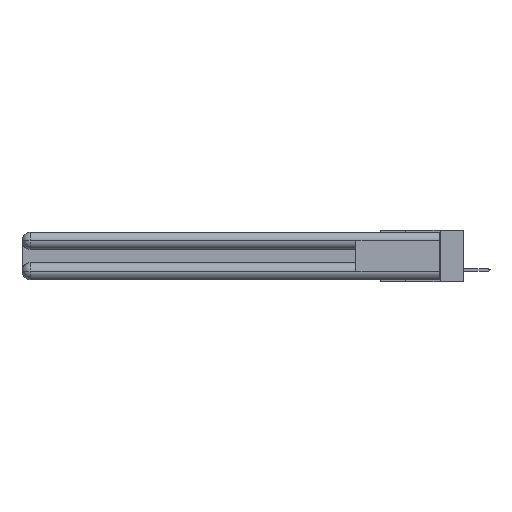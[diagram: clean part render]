
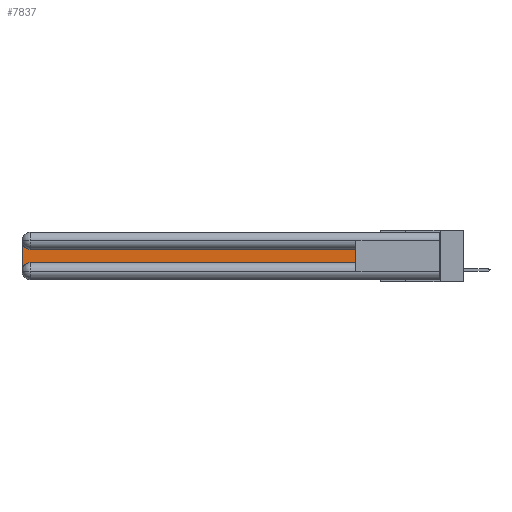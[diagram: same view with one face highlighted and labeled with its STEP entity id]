
A CAD part, left-side view. The second image highlights one B-rep face of the part: STEP entity #7837.
In plain terms, the highlighted planar face has unit normal (-1, 0, 0).
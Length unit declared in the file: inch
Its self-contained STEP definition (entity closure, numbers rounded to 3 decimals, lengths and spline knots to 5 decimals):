
#188 = EDGE_CURVE ( 'NONE', #23155, #506, #2117, .T. ) ;
#506 = VERTEX_POINT ( 'NONE', #878 ) ;
#878 = CARTESIAN_POINT ( 'NONE',  ( 0.075, 2.94, -0.2175 ) ) ;
#973 = CARTESIAN_POINT ( 'NONE',  ( 0.075, 0.6, -0.1225 ) ) ;
#992 = FACE_OUTER_BOUND ( 'NONE', #26921, .T. ) ;
#1017 = AXIS2_PLACEMENT_3D ( 'NONE', #15158, #3985, #22976 ) ;
#1837 = ORIENTED_EDGE ( 'NONE', *, *, #188, .T. ) ;
#2117 = CIRCLE ( 'NONE', #8973, 0.06 ) ;
#2458 = ORIENTED_EDGE ( 'NONE', *, *, #16512, .T. ) ;
#3915 = LINE ( 'NONE', #973, #23005 ) ;
#3985 = DIRECTION ( 'NONE',  ( 1., 0., 0. ) ) ;
#4199 = CIRCLE ( 'NONE', #1017, 0.06 ) ;
#5068 = CARTESIAN_POINT ( 'NONE',  ( 0.075, 0.6, -0.2175 ) ) ;
#6595 = CARTESIAN_POINT ( 'NONE',  ( 0.075, 3., -0.2175 ) ) ;
#7837 = ADVANCED_FACE ( 'NONE', ( #992 ), #11448, .F. ) ;
#8078 = AXIS2_PLACEMENT_3D ( 'NONE', #23175, #27730, #20929 ) ;
#8739 = VERTEX_POINT ( 'NONE', #21178 ) ;
#8973 = AXIS2_PLACEMENT_3D ( 'NONE', #25757, #11678, #11375 ) ;
#9025 = CARTESIAN_POINT ( 'NONE',  ( 0.075, 0.6, -0.1225 ) ) ;
#9515 = EDGE_CURVE ( 'NONE', #15710, #8739, #4199, .T. ) ;
#9589 = ORIENTED_EDGE ( 'NONE', *, *, #11261, .T. ) ;
#11261 = EDGE_CURVE ( 'NONE', #8739, #23155, #26998, .T. ) ;
#11375 = DIRECTION ( 'NONE',  ( 0., 0., -1. ) ) ;
#11448 = PLANE ( 'NONE',  #8078 ) ;
#11678 = DIRECTION ( 'NONE',  ( 1., 0., 0. ) ) ;
#12308 = ORIENTED_EDGE ( 'NONE', *, *, #24619, .T. ) ;
#13381 = CARTESIAN_POINT ( 'NONE',  ( 0.075, 2.94, -0.1225 ) ) ;
#13755 = VECTOR ( 'NONE', #20746, 39.37008 ) ;
#13794 = VECTOR ( 'NONE', #29493, 39.37008 ) ;
#14466 = VERTEX_POINT ( 'NONE', #5068 ) ;
#15158 = CARTESIAN_POINT ( 'NONE',  ( 0.075, 2.94, -0.0625 ) ) ;
#15416 = CARTESIAN_POINT ( 'NONE',  ( 0.075, 0.6, -0.2175 ) ) ;
#15710 = VERTEX_POINT ( 'NONE', #13381 ) ;
#15789 = ORIENTED_EDGE ( 'NONE', *, *, #26284, .T. ) ;
#16512 = EDGE_CURVE ( 'NONE', #14466, #16564, #20800, .T. ) ;
#16564 = VERTEX_POINT ( 'NONE', #9025 ) ;
#19490 = CARTESIAN_POINT ( 'NONE',  ( 0.075, 0.6, -0.2175 ) ) ;
#19597 = VECTOR ( 'NONE', #26778, 39.37008 ) ;
#19760 = DIRECTION ( 'NONE',  ( 0., 1., 0. ) ) ;
#20746 = DIRECTION ( 'NONE',  ( 0., 0., -1. ) ) ;
#20800 = LINE ( 'NONE', #15416, #13794 ) ;
#20929 = DIRECTION ( 'NONE',  ( 0., 0., -1. ) ) ;
#21178 = CARTESIAN_POINT ( 'NONE',  ( 0.075, 3., -0.0625 ) ) ;
#22976 = DIRECTION ( 'NONE',  ( 0., 0., -1. ) ) ;
#23005 = VECTOR ( 'NONE', #19760, 39.37008 ) ;
#23155 = VERTEX_POINT ( 'NONE', #25401 ) ;
#23175 = CARTESIAN_POINT ( 'NONE',  ( 0.075, 3., -0.1225 ) ) ;
#24619 = EDGE_CURVE ( 'NONE', #506, #14466, #28627, .T. ) ;
#25401 = CARTESIAN_POINT ( 'NONE',  ( 0.075, 3., -0.2775 ) ) ;
#25757 = CARTESIAN_POINT ( 'NONE',  ( 0.075, 2.94, -0.2775 ) ) ;
#26284 = EDGE_CURVE ( 'NONE', #16564, #15710, #3915, .T. ) ;
#26778 = DIRECTION ( 'NONE',  ( 0., -1., 0. ) ) ;
#26921 = EDGE_LOOP ( 'NONE', ( #15789, #29627, #9589, #1837, #12308, #2458 ) ) ;
#26998 = LINE ( 'NONE', #6595, #13755 ) ;
#27730 = DIRECTION ( 'NONE',  ( 1., 0., 0. ) ) ;
#28627 = LINE ( 'NONE', #19490, #19597 ) ;
#29493 = DIRECTION ( 'NONE',  ( 0., 0., 1. ) ) ;
#29627 = ORIENTED_EDGE ( 'NONE', *, *, #9515, .T. ) ;
